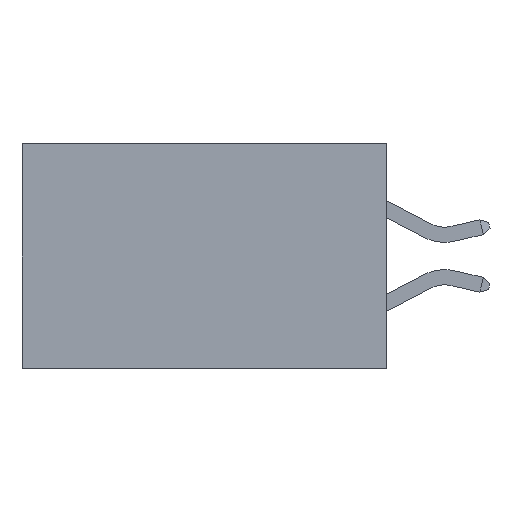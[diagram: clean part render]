
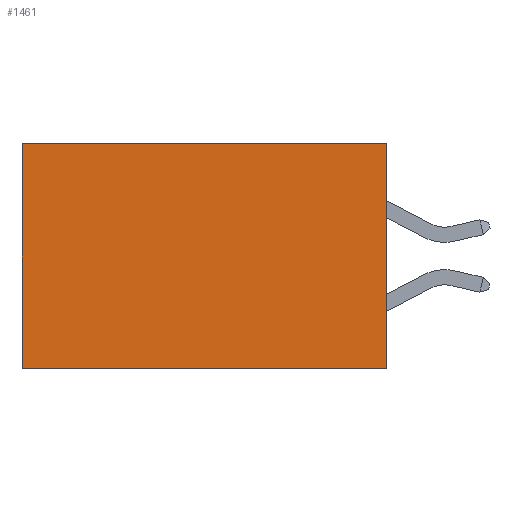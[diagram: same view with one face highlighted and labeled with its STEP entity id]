
A CAD part, left-side view. The second image highlights one B-rep face of the part: STEP entity #1461.
In plain terms, the highlighted planar face has unit normal (-1, 0, 0).
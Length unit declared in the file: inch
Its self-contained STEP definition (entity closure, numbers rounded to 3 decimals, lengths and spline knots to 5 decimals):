
#383 = DIRECTION ( 'NONE',  ( 1., 0., 0. ) ) ;
#686 = LINE ( 'NONE', #1403, #3859 ) ;
#1403 = CARTESIAN_POINT ( 'NONE',  ( 0.2615, 0., 0. ) ) ;
#1461 = ADVANCED_FACE ( 'NONE', ( #4953 ), #4382, .F. ) ;
#1487 = DIRECTION ( 'NONE',  ( 0., 1., 0. ) ) ;
#1533 = VECTOR ( 'NONE', #2024, 39.37008 ) ;
#1993 = VECTOR ( 'NONE', #5176, 39.37008 ) ;
#2024 = DIRECTION ( 'NONE',  ( 0., 1., 0. ) ) ;
#2056 = CARTESIAN_POINT ( 'NONE',  ( 0.2615, 0., -0.37 ) ) ;
#2256 = ORIENTED_EDGE ( 'NONE', *, *, #3349, .F. ) ;
#2273 = ORIENTED_EDGE ( 'NONE', *, *, #3624, .T. ) ;
#2348 = VECTOR ( 'NONE', #4898, 39.37008 ) ;
#3069 = CARTESIAN_POINT ( 'NONE',  ( 0.2615, 0.6, 0. ) ) ;
#3151 = AXIS2_PLACEMENT_3D ( 'NONE', #5050, #383, #3752 ) ;
#3349 = EDGE_CURVE ( 'NONE', #4437, #7770, #5784, .T. ) ;
#3624 = EDGE_CURVE ( 'NONE', #4437, #6276, #686, .T. ) ;
#3702 = EDGE_CURVE ( 'NONE', #7770, #4914, #4737, .T. ) ;
#3752 = DIRECTION ( 'NONE',  ( 0., 0., -1. ) ) ;
#3783 = CARTESIAN_POINT ( 'NONE',  ( 0.2615, 0., 0. ) ) ;
#3859 = VECTOR ( 'NONE', #1487, 39.37008 ) ;
#3867 = CARTESIAN_POINT ( 'NONE',  ( 0.2615, 0., -0.37 ) ) ;
#4382 = PLANE ( 'NONE',  #3151 ) ;
#4437 = VERTEX_POINT ( 'NONE', #3783 ) ;
#4737 = LINE ( 'NONE', #2056, #1533 ) ;
#4898 = DIRECTION ( 'NONE',  ( 0., 0., -1. ) ) ;
#4914 = VERTEX_POINT ( 'NONE', #6109 ) ;
#4953 = FACE_OUTER_BOUND ( 'NONE', #7342, .T. ) ;
#5050 = CARTESIAN_POINT ( 'NONE',  ( 0.2615, 0., -0.37 ) ) ;
#5165 = EDGE_CURVE ( 'NONE', #6276, #4914, #6269, .T. ) ;
#5176 = DIRECTION ( 'NONE',  ( 0., 0., -1. ) ) ;
#5784 = LINE ( 'NONE', #3867, #1993 ) ;
#6109 = CARTESIAN_POINT ( 'NONE',  ( 0.2615, 0.6, -0.37 ) ) ;
#6269 = LINE ( 'NONE', #8139, #2348 ) ;
#6276 = VERTEX_POINT ( 'NONE', #3069 ) ;
#6842 = ORIENTED_EDGE ( 'NONE', *, *, #5165, .T. ) ;
#7019 = CARTESIAN_POINT ( 'NONE',  ( 0.2615, 0., -0.37 ) ) ;
#7342 = EDGE_LOOP ( 'NONE', ( #6842, #7976, #2256, #2273 ) ) ;
#7770 = VERTEX_POINT ( 'NONE', #7019 ) ;
#7976 = ORIENTED_EDGE ( 'NONE', *, *, #3702, .F. ) ;
#8139 = CARTESIAN_POINT ( 'NONE',  ( 0.2615, 0.6, -0.37 ) ) ;
